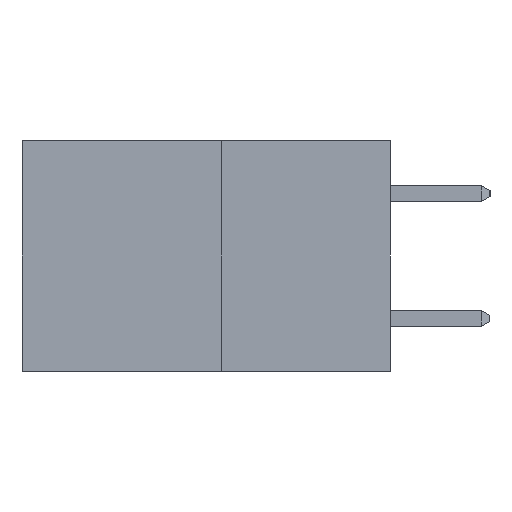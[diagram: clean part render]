
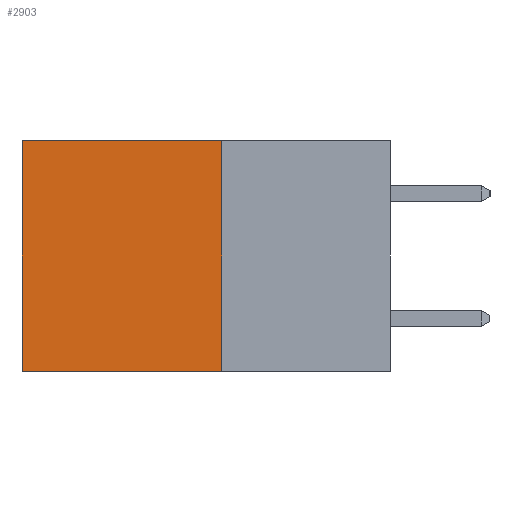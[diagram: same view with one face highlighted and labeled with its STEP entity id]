
A CAD part, left-side view. The second image highlights one B-rep face of the part: STEP entity #2903.
In plain terms, the highlighted planar face has unit normal (-1, 0, 0).
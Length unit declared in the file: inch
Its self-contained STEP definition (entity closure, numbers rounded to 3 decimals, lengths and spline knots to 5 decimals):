
#141 = CARTESIAN_POINT ( 'NONE',  ( 0.277, 0.59, 0. ) ) ;
#301 = VECTOR ( 'NONE', #9386, 39.37008 ) ;
#510 = CARTESIAN_POINT ( 'NONE',  ( 0.277, 0.27, -0.37 ) ) ;
#1362 = VERTEX_POINT ( 'NONE', #141 ) ;
#2308 = DIRECTION ( 'NONE',  ( 0., 0., -1. ) ) ;
#2668 = VERTEX_POINT ( 'NONE', #11009 ) ;
#2903 = ADVANCED_FACE ( 'NONE', ( #9252 ), #14320, .F. ) ;
#3121 = DIRECTION ( 'NONE',  ( 1., 0., 0. ) ) ;
#3454 = VERTEX_POINT ( 'NONE', #6575 ) ;
#5044 = ORIENTED_EDGE ( 'NONE', *, *, #14236, .F. ) ;
#5188 = DIRECTION ( 'NONE',  ( 0., 0., -1. ) ) ;
#5389 = EDGE_CURVE ( 'NONE', #1362, #3454, #6841, .T. ) ;
#5553 = CARTESIAN_POINT ( 'NONE',  ( 0.277, 0.27, 0. ) ) ;
#6271 = CARTESIAN_POINT ( 'NONE',  ( 0.277, 0.27, 0. ) ) ;
#6345 = DIRECTION ( 'NONE',  ( 0., 1., 0. ) ) ;
#6575 = CARTESIAN_POINT ( 'NONE',  ( 0.277, 0.59, -0.37 ) ) ;
#6841 = LINE ( 'NONE', #13157, #301 ) ;
#7496 = EDGE_CURVE ( 'NONE', #7532, #1362, #13006, .T. ) ;
#7532 = VERTEX_POINT ( 'NONE', #5553 ) ;
#8138 = LINE ( 'NONE', #510, #10756 ) ;
#8752 = ORIENTED_EDGE ( 'NONE', *, *, #7496, .T. ) ;
#9252 = FACE_OUTER_BOUND ( 'NONE', #9987, .T. ) ;
#9386 = DIRECTION ( 'NONE',  ( 0., 0., -1. ) ) ;
#9431 = CARTESIAN_POINT ( 'NONE',  ( 0.277, 0.27, -0.37 ) ) ;
#9987 = EDGE_LOOP ( 'NONE', ( #14685, #14029, #5044, #8752 ) ) ;
#10093 = DIRECTION ( 'NONE',  ( 0., 1., 0. ) ) ;
#10756 = VECTOR ( 'NONE', #10093, 39.37008 ) ;
#11009 = CARTESIAN_POINT ( 'NONE',  ( 0.277, 0.27, -0.37 ) ) ;
#11427 = EDGE_CURVE ( 'NONE', #2668, #3454, #8138, .T. ) ;
#11588 = VECTOR ( 'NONE', #2308, 39.37008 ) ;
#12668 = VECTOR ( 'NONE', #6345, 39.37008 ) ;
#13006 = LINE ( 'NONE', #6271, #12668 ) ;
#13157 = CARTESIAN_POINT ( 'NONE',  ( 0.277, 0.59, -0.37 ) ) ;
#13698 = AXIS2_PLACEMENT_3D ( 'NONE', #14454, #3121, #5188 ) ;
#14029 = ORIENTED_EDGE ( 'NONE', *, *, #11427, .F. ) ;
#14223 = LINE ( 'NONE', #9431, #11588 ) ;
#14236 = EDGE_CURVE ( 'NONE', #7532, #2668, #14223, .T. ) ;
#14320 = PLANE ( 'NONE',  #13698 ) ;
#14454 = CARTESIAN_POINT ( 'NONE',  ( 0.277, 0.27, -0.37 ) ) ;
#14685 = ORIENTED_EDGE ( 'NONE', *, *, #5389, .T. ) ;
